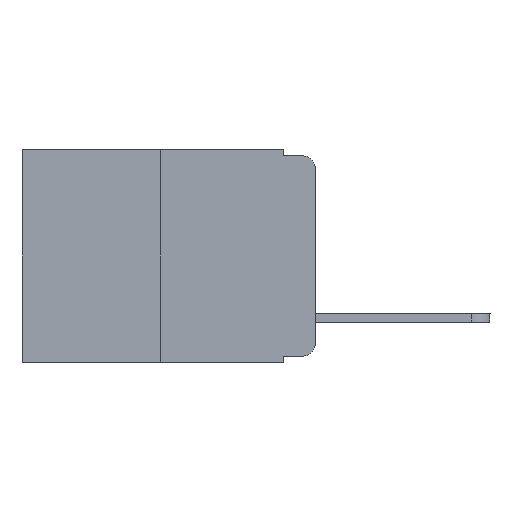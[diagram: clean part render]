
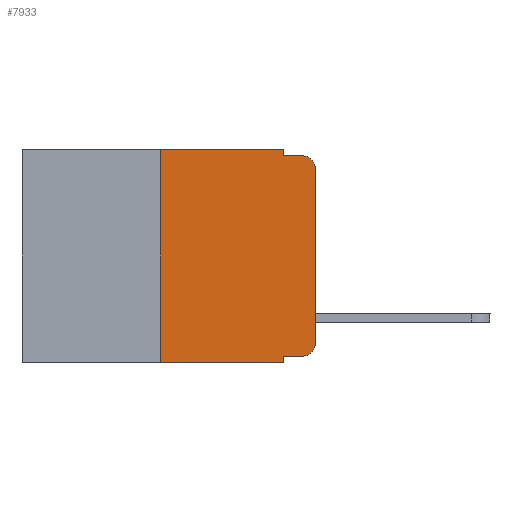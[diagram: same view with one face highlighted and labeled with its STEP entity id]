
A CAD part, left-side view. The second image highlights one B-rep face of the part: STEP entity #7933.
In plain terms, the highlighted planar face has unit normal (-1, 0, 0).
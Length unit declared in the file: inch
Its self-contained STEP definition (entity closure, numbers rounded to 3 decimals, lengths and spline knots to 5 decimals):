
#257 = DIRECTION ( 'NONE',  ( 1., 0., 0. ) ) ;
#334 = LINE ( 'NONE', #9897, #9705 ) ;
#482 = DIRECTION ( 'NONE',  ( 0., -1., 0. ) ) ;
#647 = DIRECTION ( 'NONE',  ( 0., -1., 0. ) ) ;
#663 = VERTEX_POINT ( 'NONE', #9354 ) ;
#729 = VECTOR ( 'NONE', #5422, 39.37008 ) ;
#782 = CARTESIAN_POINT ( 'NONE',  ( 0., 0.02, -0.333 ) ) ;
#1031 = ORIENTED_EDGE ( 'NONE', *, *, #10003, .T. ) ;
#1362 = DIRECTION ( 'NONE',  ( 0., -1., 0. ) ) ;
#1480 = CARTESIAN_POINT ( 'NONE',  ( 0., 0.051, -0.333 ) ) ;
#1638 = EDGE_CURVE ( 'NONE', #2856, #5619, #5467, .T. ) ;
#2058 = AXIS2_PLACEMENT_3D ( 'NONE', #3129, #2394, #7936 ) ;
#2255 = CARTESIAN_POINT ( 'NONE',  ( 0., 0., -0.313 ) ) ;
#2267 = AXIS2_PLACEMENT_3D ( 'NONE', #4896, #257, #6606 ) ;
#2309 = CARTESIAN_POINT ( 'NONE',  ( 0., 0.051, -0.01 ) ) ;
#2315 = EDGE_CURVE ( 'NONE', #5069, #6939, #5015, .T. ) ;
#2383 = AXIS2_PLACEMENT_3D ( 'NONE', #4451, #5237, #9204 ) ;
#2394 = DIRECTION ( 'NONE',  ( -1., 0., 0. ) ) ;
#2754 = CARTESIAN_POINT ( 'NONE',  ( 0., 0.051, -0.333 ) ) ;
#2782 = CARTESIAN_POINT ( 'NONE',  ( 0., 0.051, -0.01 ) ) ;
#2848 = EDGE_CURVE ( 'NONE', #9752, #6970, #4310, .T. ) ;
#2856 = VERTEX_POINT ( 'NONE', #2754 ) ;
#3129 = CARTESIAN_POINT ( 'NONE',  ( 0., 0.02, -0.313 ) ) ;
#3146 = CARTESIAN_POINT ( 'NONE',  ( 0., 0.051, -0.343 ) ) ;
#3157 = VERTEX_POINT ( 'NONE', #6854 ) ;
#3427 = VECTOR ( 'NONE', #1362, 39.37008 ) ;
#3498 = CARTESIAN_POINT ( 'NONE',  ( 0., 0.051, 0. ) ) ;
#3664 = LINE ( 'NONE', #9273, #6217 ) ;
#3880 = CARTESIAN_POINT ( 'NONE',  ( 0., 0.25, -0.343 ) ) ;
#3987 = ORIENTED_EDGE ( 'NONE', *, *, #4691, .F. ) ;
#4310 = LINE ( 'NONE', #7494, #4363 ) ;
#4363 = VECTOR ( 'NONE', #4416, 39.37008 ) ;
#4383 = CIRCLE ( 'NONE', #2058, 0.02 ) ;
#4416 = DIRECTION ( 'NONE',  ( 0., 0., -1. ) ) ;
#4451 = CARTESIAN_POINT ( 'NONE',  ( 0., 0.02, -0.03 ) ) ;
#4691 = EDGE_CURVE ( 'NONE', #2856, #6939, #5473, .T. ) ;
#4772 = ORIENTED_EDGE ( 'NONE', *, *, #1638, .T. ) ;
#4896 = CARTESIAN_POINT ( 'NONE',  ( 0., 0.473, 0. ) ) ;
#5015 = LINE ( 'NONE', #8194, #7250 ) ;
#5069 = VERTEX_POINT ( 'NONE', #3880 ) ;
#5177 = LINE ( 'NONE', #2782, #3427 ) ;
#5237 = DIRECTION ( 'NONE',  ( -1., 0., 0. ) ) ;
#5314 = ORIENTED_EDGE ( 'NONE', *, *, #9378, .T. ) ;
#5422 = DIRECTION ( 'NONE',  ( 0., 0., -1. ) ) ;
#5467 = LINE ( 'NONE', #1480, #7100 ) ;
#5473 = LINE ( 'NONE', #10164, #729 ) ;
#5539 = EDGE_CURVE ( 'NONE', #5069, #6857, #3664, .T. ) ;
#5604 = ORIENTED_EDGE ( 'NONE', *, *, #9365, .F. ) ;
#5619 = VERTEX_POINT ( 'NONE', #782 ) ;
#5663 = ORIENTED_EDGE ( 'NONE', *, *, #2315, .T. ) ;
#6209 = CARTESIAN_POINT ( 'NONE',  ( 0., 0.473, 0. ) ) ;
#6217 = VECTOR ( 'NONE', #7585, 39.37008 ) ;
#6606 = DIRECTION ( 'NONE',  ( 0., 0., -1. ) ) ;
#6854 = CARTESIAN_POINT ( 'NONE',  ( 0., 0., -0.03 ) ) ;
#6857 = VERTEX_POINT ( 'NONE', #8432 ) ;
#6883 = CIRCLE ( 'NONE', #2383, 0.02 ) ;
#6939 = VERTEX_POINT ( 'NONE', #3146 ) ;
#6970 = VERTEX_POINT ( 'NONE', #2309 ) ;
#7100 = VECTOR ( 'NONE', #647, 39.37008 ) ;
#7250 = VECTOR ( 'NONE', #7417, 39.37008 ) ;
#7392 = DIRECTION ( 'NONE',  ( 0., 0., 1. ) ) ;
#7417 = DIRECTION ( 'NONE',  ( 0., -1., 0. ) ) ;
#7494 = CARTESIAN_POINT ( 'NONE',  ( 0., 0.051, 0. ) ) ;
#7542 = VECTOR ( 'NONE', #482, 39.37008 ) ;
#7585 = DIRECTION ( 'NONE',  ( 0., 0., 1. ) ) ;
#7906 = ORIENTED_EDGE ( 'NONE', *, *, #2848, .F. ) ;
#7933 = ADVANCED_FACE ( 'NONE', ( #8864 ), #8082, .F. ) ;
#7936 = DIRECTION ( 'NONE',  ( 0., 0., -1. ) ) ;
#8082 = PLANE ( 'NONE',  #2267 ) ;
#8122 = EDGE_CURVE ( 'NONE', #6970, #663, #5177, .T. ) ;
#8194 = CARTESIAN_POINT ( 'NONE',  ( 0., 0.473, -0.343 ) ) ;
#8337 = EDGE_LOOP ( 'NONE', ( #9458, #5314, #8449, #7906, #5604, #9943, #5663, #3987, #4772, #1031 ) ) ;
#8425 = LINE ( 'NONE', #6209, #7542 ) ;
#8432 = CARTESIAN_POINT ( 'NONE',  ( 0., 0.25, 0. ) ) ;
#8449 = ORIENTED_EDGE ( 'NONE', *, *, #8122, .F. ) ;
#8864 = FACE_OUTER_BOUND ( 'NONE', #8337, .T. ) ;
#8873 = EDGE_CURVE ( 'NONE', #9411, #3157, #334, .T. ) ;
#9204 = DIRECTION ( 'NONE',  ( 0., 0., -1. ) ) ;
#9273 = CARTESIAN_POINT ( 'NONE',  ( 0., 0.25, 0. ) ) ;
#9354 = CARTESIAN_POINT ( 'NONE',  ( 0., 0.02, -0.01 ) ) ;
#9365 = EDGE_CURVE ( 'NONE', #6857, #9752, #8425, .T. ) ;
#9378 = EDGE_CURVE ( 'NONE', #3157, #663, #6883, .T. ) ;
#9411 = VERTEX_POINT ( 'NONE', #2255 ) ;
#9458 = ORIENTED_EDGE ( 'NONE', *, *, #8873, .T. ) ;
#9705 = VECTOR ( 'NONE', #7392, 39.37008 ) ;
#9752 = VERTEX_POINT ( 'NONE', #3498 ) ;
#9897 = CARTESIAN_POINT ( 'NONE',  ( 0., 0., 0. ) ) ;
#9943 = ORIENTED_EDGE ( 'NONE', *, *, #5539, .F. ) ;
#10003 = EDGE_CURVE ( 'NONE', #5619, #9411, #4383, .T. ) ;
#10164 = CARTESIAN_POINT ( 'NONE',  ( 0., 0.051, 0. ) ) ;
